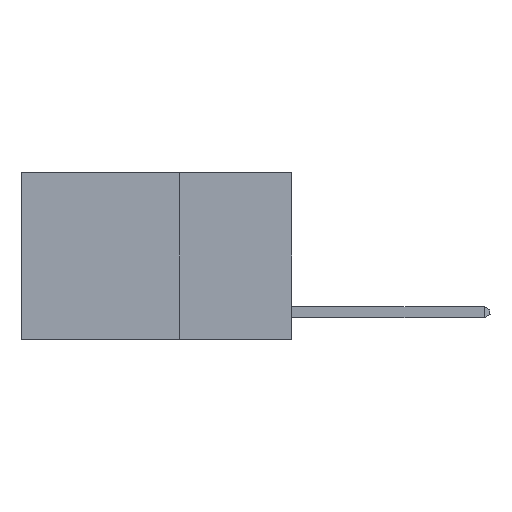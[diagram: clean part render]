
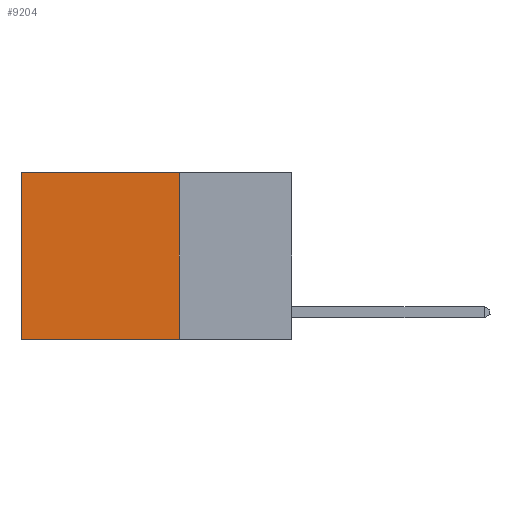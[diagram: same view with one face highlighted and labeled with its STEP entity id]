
A CAD part, left-side view. The second image highlights one B-rep face of the part: STEP entity #9204.
In plain terms, the highlighted planar face has unit normal (-1, 0, 0).
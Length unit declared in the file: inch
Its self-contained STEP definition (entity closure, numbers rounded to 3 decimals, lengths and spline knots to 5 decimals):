
#343 = CARTESIAN_POINT ( 'NONE',  ( 0.2625, 0.6, -0.37 ) ) ;
#2514 = EDGE_LOOP ( 'NONE', ( #17387, #10290, #18246, #7054 ) ) ;
#3383 = LINE ( 'NONE', #5934, #16630 ) ;
#3634 = VERTEX_POINT ( 'NONE', #12131 ) ;
#3928 = EDGE_CURVE ( 'NONE', #3634, #11330, #19722, .T. ) ;
#4965 = LINE ( 'NONE', #8009, #18726 ) ;
#5627 = FACE_OUTER_BOUND ( 'NONE', #2514, .T. ) ;
#5755 = VERTEX_POINT ( 'NONE', #9264 ) ;
#5934 = CARTESIAN_POINT ( 'NONE',  ( 0.2625, 0.25, 0. ) ) ;
#6004 = DIRECTION ( 'NONE',  ( 0., 1., 0. ) ) ;
#7054 = ORIENTED_EDGE ( 'NONE', *, *, #10841, .T. ) ;
#8009 = CARTESIAN_POINT ( 'NONE',  ( 0.2625, 0.6, 0. ) ) ;
#8955 = DIRECTION ( 'NONE',  ( 0., 0., -1. ) ) ;
#9204 = ADVANCED_FACE ( 'NONE', ( #5627 ), #19527, .F. ) ;
#9264 = CARTESIAN_POINT ( 'NONE',  ( 0.2625, 0.6, 0. ) ) ;
#9267 = DIRECTION ( 'NONE',  ( 1., 0., 0. ) ) ;
#9489 = DIRECTION ( 'NONE',  ( 0., 1., 0. ) ) ;
#10290 = ORIENTED_EDGE ( 'NONE', *, *, #3928, .F. ) ;
#10841 = EDGE_CURVE ( 'NONE', #19247, #5755, #3383, .T. ) ;
#10922 = CARTESIAN_POINT ( 'NONE',  ( 0.2625, 0.25, 0. ) ) ;
#11159 = VECTOR ( 'NONE', #9489, 39.37008 ) ;
#11285 = EDGE_CURVE ( 'NONE', #19247, #3634, #16613, .T. ) ;
#11330 = VERTEX_POINT ( 'NONE', #343 ) ;
#12056 = VECTOR ( 'NONE', #8955, 39.37008 ) ;
#12131 = CARTESIAN_POINT ( 'NONE',  ( 0.2625, 0.25, -0.37 ) ) ;
#12334 = CARTESIAN_POINT ( 'NONE',  ( 0.2625, 0.25, 0. ) ) ;
#13389 = AXIS2_PLACEMENT_3D ( 'NONE', #10922, #9267, #21268 ) ;
#16613 = LINE ( 'NONE', #12334, #12056 ) ;
#16630 = VECTOR ( 'NONE', #6004, 39.37008 ) ;
#17387 = ORIENTED_EDGE ( 'NONE', *, *, #18505, .T. ) ;
#18246 = ORIENTED_EDGE ( 'NONE', *, *, #11285, .F. ) ;
#18505 = EDGE_CURVE ( 'NONE', #5755, #11330, #4965, .T. ) ;
#18726 = VECTOR ( 'NONE', #20019, 39.37008 ) ;
#19247 = VERTEX_POINT ( 'NONE', #21424 ) ;
#19527 = PLANE ( 'NONE',  #13389 ) ;
#19722 = LINE ( 'NONE', #19743, #11159 ) ;
#19743 = CARTESIAN_POINT ( 'NONE',  ( 0.2625, 0.25, -0.37 ) ) ;
#20019 = DIRECTION ( 'NONE',  ( 0., 0., -1. ) ) ;
#21268 = DIRECTION ( 'NONE',  ( 0., 0., -1. ) ) ;
#21424 = CARTESIAN_POINT ( 'NONE',  ( 0.2625, 0.25, 0. ) ) ;
